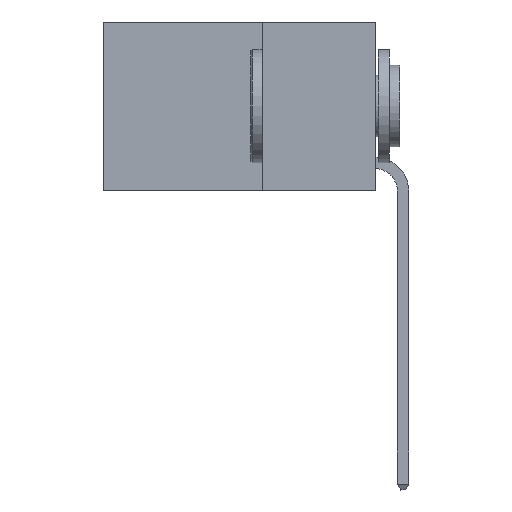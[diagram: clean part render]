
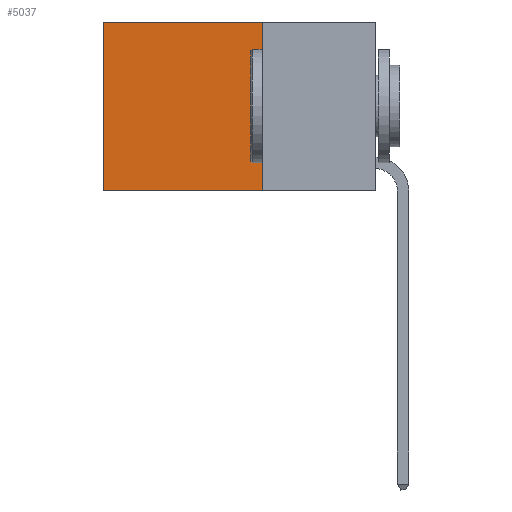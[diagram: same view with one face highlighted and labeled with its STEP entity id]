
A CAD part, left-side view. The second image highlights one B-rep face of the part: STEP entity #5037.
In plain terms, the highlighted planar face has unit normal (-1, 0, 0).
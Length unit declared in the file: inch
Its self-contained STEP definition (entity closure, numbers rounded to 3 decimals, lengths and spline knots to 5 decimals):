
#113 = VERTEX_POINT ( 'NONE', #852 ) ;
#290 = LINE ( 'NONE', #9215, #7395 ) ;
#639 = CARTESIAN_POINT ( 'NONE',  ( 0.2625, 0.25, 0. ) ) ;
#852 = CARTESIAN_POINT ( 'NONE',  ( 0.2625, 0.6, 0. ) ) ;
#1119 = EDGE_CURVE ( 'NONE', #113, #9417, #6172, .T. ) ;
#1803 = LINE ( 'NONE', #5313, #8173 ) ;
#2471 = VECTOR ( 'NONE', #10442, 39.37008 ) ;
#3500 = DIRECTION ( 'NONE',  ( 0., 0., -1. ) ) ;
#3609 = EDGE_LOOP ( 'NONE', ( #5357, #5951, #9144, #9259 ) ) ;
#3665 = CARTESIAN_POINT ( 'NONE',  ( 0.2625, 0.25, 0. ) ) ;
#4456 = CARTESIAN_POINT ( 'NONE',  ( 0.2625, 0.25, 0. ) ) ;
#5037 = ADVANCED_FACE ( 'NONE', ( #11517 ), #5206, .F. ) ;
#5062 = LINE ( 'NONE', #4456, #2471 ) ;
#5089 = CARTESIAN_POINT ( 'NONE',  ( 0.2625, 0.25, -0.37 ) ) ;
#5106 = EDGE_CURVE ( 'NONE', #9341, #113, #290, .T. ) ;
#5206 = PLANE ( 'NONE',  #6081 ) ;
#5313 = CARTESIAN_POINT ( 'NONE',  ( 0.2625, 0.25, -0.37 ) ) ;
#5357 = ORIENTED_EDGE ( 'NONE', *, *, #1119, .T. ) ;
#5670 = DIRECTION ( 'NONE',  ( 0., 1., 0. ) ) ;
#5951 = ORIENTED_EDGE ( 'NONE', *, *, #9164, .F. ) ;
#6081 = AXIS2_PLACEMENT_3D ( 'NONE', #639, #7070, #11469 ) ;
#6172 = LINE ( 'NONE', #11629, #11160 ) ;
#7070 = DIRECTION ( 'NONE',  ( 1., 0., 0. ) ) ;
#7200 = DIRECTION ( 'NONE',  ( 0., 1., 0. ) ) ;
#7395 = VECTOR ( 'NONE', #5670, 39.37008 ) ;
#8070 = VERTEX_POINT ( 'NONE', #5089 ) ;
#8173 = VECTOR ( 'NONE', #7200, 39.37008 ) ;
#8910 = EDGE_CURVE ( 'NONE', #9341, #8070, #5062, .T. ) ;
#9144 = ORIENTED_EDGE ( 'NONE', *, *, #8910, .F. ) ;
#9164 = EDGE_CURVE ( 'NONE', #8070, #9417, #1803, .T. ) ;
#9215 = CARTESIAN_POINT ( 'NONE',  ( 0.2625, 0.25, 0. ) ) ;
#9259 = ORIENTED_EDGE ( 'NONE', *, *, #5106, .T. ) ;
#9341 = VERTEX_POINT ( 'NONE', #3665 ) ;
#9417 = VERTEX_POINT ( 'NONE', #9918 ) ;
#9918 = CARTESIAN_POINT ( 'NONE',  ( 0.2625, 0.6, -0.37 ) ) ;
#10442 = DIRECTION ( 'NONE',  ( 0., 0., -1. ) ) ;
#11160 = VECTOR ( 'NONE', #3500, 39.37008 ) ;
#11469 = DIRECTION ( 'NONE',  ( 0., 0., -1. ) ) ;
#11517 = FACE_OUTER_BOUND ( 'NONE', #3609, .T. ) ;
#11629 = CARTESIAN_POINT ( 'NONE',  ( 0.2625, 0.6, 0. ) ) ;
